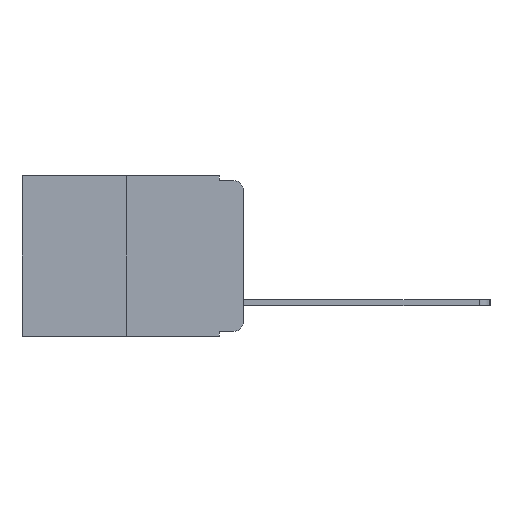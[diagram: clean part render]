
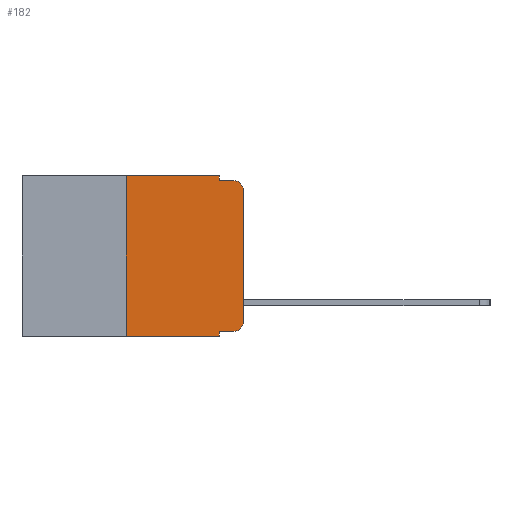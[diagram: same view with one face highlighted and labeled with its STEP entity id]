
A CAD part, left-side view. The second image highlights one B-rep face of the part: STEP entity #182.
In plain terms, the highlighted planar face has unit normal (-1, 0, 0).
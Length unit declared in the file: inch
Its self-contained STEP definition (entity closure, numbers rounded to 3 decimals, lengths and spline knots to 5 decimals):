
#182 = ADVANCED_FACE ( 'NONE', ( #2165 ), #13003, .F. ) ;
#273 = CARTESIAN_POINT ( 'NONE',  ( 0., 0.051, -0.01 ) ) ;
#582 = CARTESIAN_POINT ( 'NONE',  ( 0., 0.02, -0.01 ) ) ;
#944 = DIRECTION ( 'NONE',  ( 1., 0., 0. ) ) ;
#966 = VERTEX_POINT ( 'NONE', #4547 ) ;
#1314 = VERTEX_POINT ( 'NONE', #4642 ) ;
#1515 = CARTESIAN_POINT ( 'NONE',  ( 0., 0., 0. ) ) ;
#1976 = VERTEX_POINT ( 'NONE', #6510 ) ;
#2020 = EDGE_LOOP ( 'NONE', ( #6297, #8055, #3915, #14797, #14811, #3321, #3722, #12953, #12105, #3197 ) ) ;
#2028 = CARTESIAN_POINT ( 'NONE',  ( 0., 0.473, 0. ) ) ;
#2165 = FACE_OUTER_BOUND ( 'NONE', #2020, .T. ) ;
#2551 = VERTEX_POINT ( 'NONE', #14128 ) ;
#2787 = DIRECTION ( 'NONE',  ( 0., 0., 1. ) ) ;
#3111 = AXIS2_PLACEMENT_3D ( 'NONE', #5972, #13745, #7085 ) ;
#3197 = ORIENTED_EDGE ( 'NONE', *, *, #6535, .T. ) ;
#3271 = CIRCLE ( 'NONE', #3111, 0.02 ) ;
#3321 = ORIENTED_EDGE ( 'NONE', *, *, #9524, .F. ) ;
#3449 = VECTOR ( 'NONE', #11812, 39.37008 ) ;
#3592 = LINE ( 'NONE', #7887, #9704 ) ;
#3722 = ORIENTED_EDGE ( 'NONE', *, *, #9913, .T. ) ;
#3915 = ORIENTED_EDGE ( 'NONE', *, *, #11727, .F. ) ;
#4547 = CARTESIAN_POINT ( 'NONE',  ( 0., 0., -0.03 ) ) ;
#4562 = LINE ( 'NONE', #9505, #10195 ) ;
#4642 = CARTESIAN_POINT ( 'NONE',  ( 0., 0.02, -0.333 ) ) ;
#5115 = VERTEX_POINT ( 'NONE', #12623 ) ;
#5380 = CARTESIAN_POINT ( 'NONE',  ( 0., 0.051, -0.343 ) ) ;
#5620 = VERTEX_POINT ( 'NONE', #13514 ) ;
#5718 = VECTOR ( 'NONE', #14336, 39.37008 ) ;
#5838 = DIRECTION ( 'NONE',  ( -1., 0., 0. ) ) ;
#5972 = CARTESIAN_POINT ( 'NONE',  ( 0., 0.02, -0.03 ) ) ;
#6001 = VECTOR ( 'NONE', #8626, 39.37008 ) ;
#6046 = VERTEX_POINT ( 'NONE', #5380 ) ;
#6234 = CARTESIAN_POINT ( 'NONE',  ( 0., 0.051, -0.333 ) ) ;
#6297 = ORIENTED_EDGE ( 'NONE', *, *, #14910, .T. ) ;
#6510 = CARTESIAN_POINT ( 'NONE',  ( 0., 0.25, -0.343 ) ) ;
#6535 = EDGE_CURVE ( 'NONE', #1314, #10278, #8356, .T. ) ;
#6566 = CARTESIAN_POINT ( 'NONE',  ( 0., 0.051, 0. ) ) ;
#6609 = LINE ( 'NONE', #6234, #3449 ) ;
#6722 = LINE ( 'NONE', #7544, #12278 ) ;
#7085 = DIRECTION ( 'NONE',  ( 0., 0., -1. ) ) ;
#7463 = CARTESIAN_POINT ( 'NONE',  ( 0., 0.25, 0. ) ) ;
#7544 = CARTESIAN_POINT ( 'NONE',  ( 0., 0.473, -0.343 ) ) ;
#7887 = CARTESIAN_POINT ( 'NONE',  ( 0., 0.25, 0. ) ) ;
#8031 = EDGE_CURVE ( 'NONE', #2551, #1314, #6609, .T. ) ;
#8055 = ORIENTED_EDGE ( 'NONE', *, *, #13977, .T. ) ;
#8196 = LINE ( 'NONE', #1515, #13748 ) ;
#8356 = CIRCLE ( 'NONE', #11773, 0.02 ) ;
#8626 = DIRECTION ( 'NONE',  ( 0., -1., 0. ) ) ;
#8790 = EDGE_CURVE ( 'NONE', #2551, #6046, #13888, .T. ) ;
#9275 = VERTEX_POINT ( 'NONE', #7463 ) ;
#9293 = CARTESIAN_POINT ( 'NONE',  ( 0., 0., -0.313 ) ) ;
#9505 = CARTESIAN_POINT ( 'NONE',  ( 0., 0.051, 0. ) ) ;
#9524 = EDGE_CURVE ( 'NONE', #1976, #9275, #3592, .T. ) ;
#9704 = VECTOR ( 'NONE', #14526, 39.37008 ) ;
#9913 = EDGE_CURVE ( 'NONE', #1976, #6046, #6722, .T. ) ;
#10149 = AXIS2_PLACEMENT_3D ( 'NONE', #2028, #944, #14851 ) ;
#10195 = VECTOR ( 'NONE', #12856, 39.37008 ) ;
#10278 = VERTEX_POINT ( 'NONE', #9293 ) ;
#10999 = EDGE_CURVE ( 'NONE', #5620, #5115, #4562, .T. ) ;
#11565 = EDGE_CURVE ( 'NONE', #9275, #5620, #14001, .T. ) ;
#11727 = EDGE_CURVE ( 'NONE', #5115, #14440, #14512, .T. ) ;
#11773 = AXIS2_PLACEMENT_3D ( 'NONE', #12508, #5838, #13608 ) ;
#11812 = DIRECTION ( 'NONE',  ( 0., -1., 0. ) ) ;
#11904 = CARTESIAN_POINT ( 'NONE',  ( 0., 0.473, 0. ) ) ;
#12105 = ORIENTED_EDGE ( 'NONE', *, *, #8031, .T. ) ;
#12278 = VECTOR ( 'NONE', #14196, 39.37008 ) ;
#12508 = CARTESIAN_POINT ( 'NONE',  ( 0., 0.02, -0.313 ) ) ;
#12623 = CARTESIAN_POINT ( 'NONE',  ( 0., 0.051, -0.01 ) ) ;
#12856 = DIRECTION ( 'NONE',  ( 0., 0., -1. ) ) ;
#12953 = ORIENTED_EDGE ( 'NONE', *, *, #8790, .F. ) ;
#13003 = PLANE ( 'NONE',  #10149 ) ;
#13046 = DIRECTION ( 'NONE',  ( 0., -1., 0. ) ) ;
#13514 = CARTESIAN_POINT ( 'NONE',  ( 0., 0.051, 0. ) ) ;
#13608 = DIRECTION ( 'NONE',  ( 0., 0., -1. ) ) ;
#13657 = VECTOR ( 'NONE', #13046, 39.37008 ) ;
#13745 = DIRECTION ( 'NONE',  ( -1., 0., 0. ) ) ;
#13748 = VECTOR ( 'NONE', #2787, 39.37008 ) ;
#13888 = LINE ( 'NONE', #6566, #5718 ) ;
#13977 = EDGE_CURVE ( 'NONE', #966, #14440, #3271, .T. ) ;
#14001 = LINE ( 'NONE', #11904, #13657 ) ;
#14128 = CARTESIAN_POINT ( 'NONE',  ( 0., 0.051, -0.333 ) ) ;
#14196 = DIRECTION ( 'NONE',  ( 0., -1., 0. ) ) ;
#14336 = DIRECTION ( 'NONE',  ( 0., 0., -1. ) ) ;
#14440 = VERTEX_POINT ( 'NONE', #582 ) ;
#14512 = LINE ( 'NONE', #273, #6001 ) ;
#14526 = DIRECTION ( 'NONE',  ( 0., 0., 1. ) ) ;
#14797 = ORIENTED_EDGE ( 'NONE', *, *, #10999, .F. ) ;
#14811 = ORIENTED_EDGE ( 'NONE', *, *, #11565, .F. ) ;
#14851 = DIRECTION ( 'NONE',  ( 0., 0., -1. ) ) ;
#14910 = EDGE_CURVE ( 'NONE', #10278, #966, #8196, .T. ) ;
